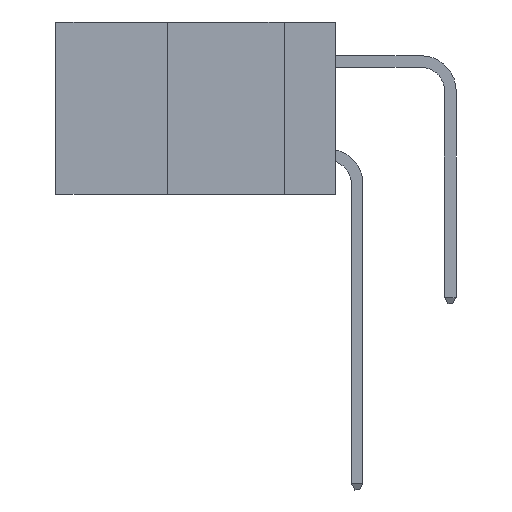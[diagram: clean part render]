
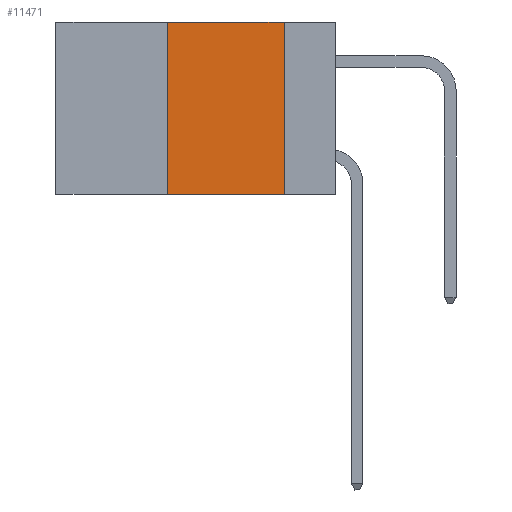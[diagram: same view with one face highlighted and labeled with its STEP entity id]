
A CAD part, left-side view. The second image highlights one B-rep face of the part: STEP entity #11471.
In plain terms, the highlighted planar face has unit normal (-1, 0, 0).
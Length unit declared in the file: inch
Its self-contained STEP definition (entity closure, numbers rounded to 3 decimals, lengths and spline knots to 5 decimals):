
#216 = DIRECTION ( 'NONE',  ( 0., -1., 0. ) ) ;
#943 = PLANE ( 'NONE',  #20248 ) ;
#1126 = EDGE_CURVE ( 'NONE', #21419, #11732, #10284, .T. ) ;
#3342 = CARTESIAN_POINT ( 'NONE',  ( 0., 0.36, 0. ) ) ;
#3467 = LINE ( 'NONE', #3342, #5295 ) ;
#3876 = EDGE_CURVE ( 'NONE', #21419, #18471, #3467, .T. ) ;
#4973 = ORIENTED_EDGE ( 'NONE', *, *, #3876, .F. ) ;
#5295 = VECTOR ( 'NONE', #18085, 39.37008 ) ;
#6162 = DIRECTION ( 'NONE',  ( 1., 0., 0. ) ) ;
#9085 = CARTESIAN_POINT ( 'NONE',  ( 0., 0.11, 0. ) ) ;
#10139 = VECTOR ( 'NONE', #216, 39.37008 ) ;
#10284 = LINE ( 'NONE', #19097, #15933 ) ;
#11118 = LINE ( 'NONE', #9085, #17564 ) ;
#11401 = CARTESIAN_POINT ( 'NONE',  ( 0., 0.6, 0. ) ) ;
#11471 = ADVANCED_FACE ( 'NONE', ( #20687 ), #943, .F. ) ;
#11606 = EDGE_LOOP ( 'NONE', ( #16120, #16589, #4973, #23121 ) ) ;
#11732 = VERTEX_POINT ( 'NONE', #12885 ) ;
#12658 = DIRECTION ( 'NONE',  ( 0., 0., -1. ) ) ;
#12885 = CARTESIAN_POINT ( 'NONE',  ( 0., 0.11, -0.37 ) ) ;
#13477 = EDGE_CURVE ( 'NONE', #17443, #11732, #11118, .T. ) ;
#13705 = CARTESIAN_POINT ( 'NONE',  ( 0., 0.11, 0. ) ) ;
#14558 = CARTESIAN_POINT ( 'NONE',  ( 0., 0.36, 0. ) ) ;
#15041 = CARTESIAN_POINT ( 'NONE',  ( 0., 0.6, 0. ) ) ;
#15933 = VECTOR ( 'NONE', #22774, 39.37008 ) ;
#16120 = ORIENTED_EDGE ( 'NONE', *, *, #13477, .F. ) ;
#16589 = ORIENTED_EDGE ( 'NONE', *, *, #20381, .F. ) ;
#16907 = CARTESIAN_POINT ( 'NONE',  ( 0., 0.36, -0.37 ) ) ;
#17443 = VERTEX_POINT ( 'NONE', #13705 ) ;
#17564 = VECTOR ( 'NONE', #12658, 39.37008 ) ;
#18085 = DIRECTION ( 'NONE',  ( 0., 0., 1. ) ) ;
#18471 = VERTEX_POINT ( 'NONE', #14558 ) ;
#19097 = CARTESIAN_POINT ( 'NONE',  ( 0., 0.6, -0.37 ) ) ;
#20248 = AXIS2_PLACEMENT_3D ( 'NONE', #11401, #6162, #20919 ) ;
#20381 = EDGE_CURVE ( 'NONE', #18471, #17443, #22204, .T. ) ;
#20687 = FACE_OUTER_BOUND ( 'NONE', #11606, .T. ) ;
#20919 = DIRECTION ( 'NONE',  ( 0., 0., -1. ) ) ;
#21419 = VERTEX_POINT ( 'NONE', #16907 ) ;
#22204 = LINE ( 'NONE', #15041, #10139 ) ;
#22774 = DIRECTION ( 'NONE',  ( 0., -1., 0. ) ) ;
#23121 = ORIENTED_EDGE ( 'NONE', *, *, #1126, .T. ) ;
